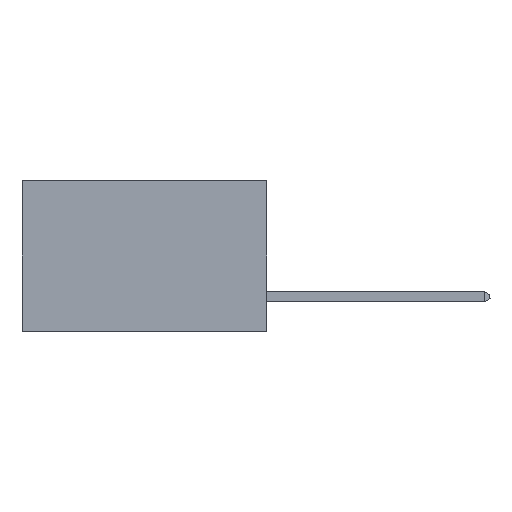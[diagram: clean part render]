
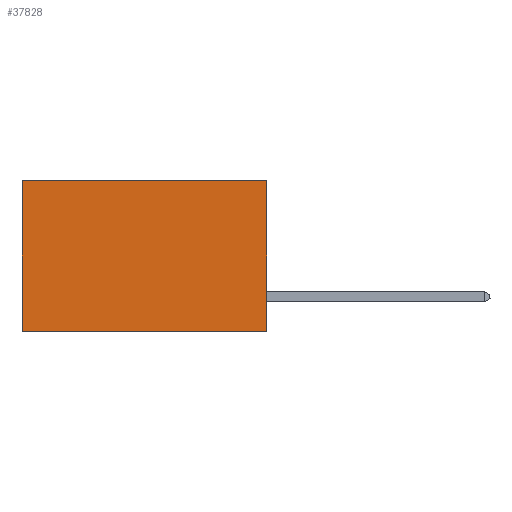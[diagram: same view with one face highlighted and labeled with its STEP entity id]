
A CAD part, left-side view. The second image highlights one B-rep face of the part: STEP entity #37828.
In plain terms, the highlighted planar face has unit normal (-1, 0, 0).
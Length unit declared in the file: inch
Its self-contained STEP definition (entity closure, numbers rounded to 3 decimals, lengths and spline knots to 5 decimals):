
#30 = VERTEX_POINT ( 'NONE', #36495 ) ;
#53 = PLANE ( 'NONE',  #33142 ) ;
#811 = FACE_OUTER_BOUND ( 'NONE', #34959, .T. ) ;
#844 = VERTEX_POINT ( 'NONE', #13918 ) ;
#1707 = CARTESIAN_POINT ( 'NONE',  ( 0.2875, 0.6, 0. ) ) ;
#2618 = DIRECTION ( 'NONE',  ( 0., 0., -1. ) ) ;
#3775 = LINE ( 'NONE', #1707, #34597 ) ;
#4311 = LINE ( 'NONE', #33484, #37021 ) ;
#4958 = VECTOR ( 'NONE', #2618, 39.37008 ) ;
#6287 = LINE ( 'NONE', #9493, #11443 ) ;
#6335 = LINE ( 'NONE', #23266, #4958 ) ;
#8974 = CARTESIAN_POINT ( 'NONE',  ( 0.2875, 0., 0. ) ) ;
#9493 = CARTESIAN_POINT ( 'NONE',  ( 0.2875, 0., -0.37 ) ) ;
#9864 = DIRECTION ( 'NONE',  ( 0., 1., 0. ) ) ;
#10899 = EDGE_CURVE ( 'NONE', #844, #21491, #6287, .T. ) ;
#11443 = VECTOR ( 'NONE', #18099, 39.37008 ) ;
#13880 = DIRECTION ( 'NONE',  ( 0., 0., -1. ) ) ;
#13918 = CARTESIAN_POINT ( 'NONE',  ( 0.2875, 0., -0.37 ) ) ;
#14164 = ORIENTED_EDGE ( 'NONE', *, *, #10899, .F. ) ;
#18099 = DIRECTION ( 'NONE',  ( 0., 1., 0. ) ) ;
#18776 = EDGE_CURVE ( 'NONE', #21471, #30, #4311, .T. ) ;
#19645 = EDGE_CURVE ( 'NONE', #30, #21491, #3775, .T. ) ;
#20901 = ORIENTED_EDGE ( 'NONE', *, *, #19645, .T. ) ;
#21401 = ORIENTED_EDGE ( 'NONE', *, *, #31748, .F. ) ;
#21471 = VERTEX_POINT ( 'NONE', #8974 ) ;
#21491 = VERTEX_POINT ( 'NONE', #35734 ) ;
#23266 = CARTESIAN_POINT ( 'NONE',  ( 0.2875, 0., 0. ) ) ;
#23981 = DIRECTION ( 'NONE',  ( 1., 0., 0. ) ) ;
#26865 = DIRECTION ( 'NONE',  ( 0., 0., -1. ) ) ;
#27238 = CARTESIAN_POINT ( 'NONE',  ( 0.2875, 0., 0. ) ) ;
#31748 = EDGE_CURVE ( 'NONE', #21471, #844, #6335, .T. ) ;
#33142 = AXIS2_PLACEMENT_3D ( 'NONE', #27238, #23981, #26865 ) ;
#33484 = CARTESIAN_POINT ( 'NONE',  ( 0.2875, 0., 0. ) ) ;
#34597 = VECTOR ( 'NONE', #13880, 39.37008 ) ;
#34959 = EDGE_LOOP ( 'NONE', ( #20901, #14164, #21401, #38428 ) ) ;
#35734 = CARTESIAN_POINT ( 'NONE',  ( 0.2875, 0.6, -0.37 ) ) ;
#36495 = CARTESIAN_POINT ( 'NONE',  ( 0.2875, 0.6, 0. ) ) ;
#37021 = VECTOR ( 'NONE', #9864, 39.37008 ) ;
#37828 = ADVANCED_FACE ( 'NONE', ( #811 ), #53, .F. ) ;
#38428 = ORIENTED_EDGE ( 'NONE', *, *, #18776, .T. ) ;
